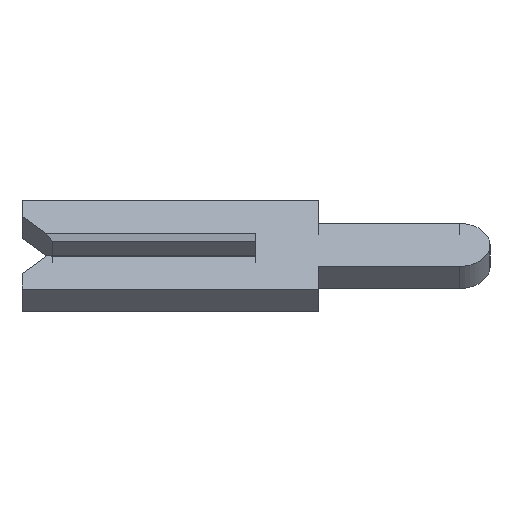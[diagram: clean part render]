
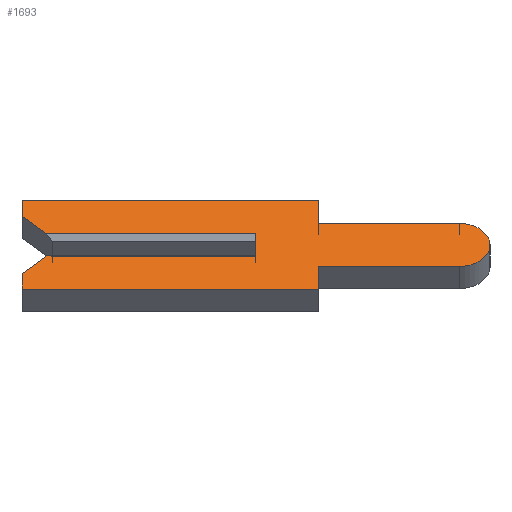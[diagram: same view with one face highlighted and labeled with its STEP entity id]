
A CAD part, left-side view. The second image highlights one B-rep face of the part: STEP entity #1693.
In plain terms, the highlighted face is planar.
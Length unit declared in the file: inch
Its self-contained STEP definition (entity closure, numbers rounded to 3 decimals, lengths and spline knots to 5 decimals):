
#19 = ORIENTED_EDGE ( 'NONE', *, *, #1580, .F. ) ;
#37 = LINE ( 'NONE', #1567, #1679 ) ;
#67 = ORIENTED_EDGE ( 'NONE', *, *, #1382, .F. ) ;
#69 = DIRECTION ( 'NONE',  ( 0., -1., 0. ) ) ;
#85 = VECTOR ( 'NONE', #317, 39.37008 ) ;
#98 = VERTEX_POINT ( 'NONE', #1309 ) ;
#99 = EDGE_CURVE ( 'NONE', #836, #1227, #289, .T. ) ;
#111 = VECTOR ( 'NONE', #650, 39.37008 ) ;
#124 = AXIS2_PLACEMENT_3D ( 'NONE', #1443, #1590, #241 ) ;
#133 = LINE ( 'NONE', #890, #406 ) ;
#152 = VECTOR ( 'NONE', #379, 39.37008 ) ;
#157 = CARTESIAN_POINT ( 'NONE',  ( -0.01, 0.15, -0.04 ) ) ;
#184 = LINE ( 'NONE', #938, #1361 ) ;
#218 = CARTESIAN_POINT ( 'NONE',  ( -0.01, 0.15, 0.04 ) ) ;
#241 = DIRECTION ( 'NONE',  ( 0., 0., -1. ) ) ;
#289 = LINE ( 'NONE', #1005, #1792 ) ;
#302 = VERTEX_POINT ( 'NONE', #1353 ) ;
#317 = DIRECTION ( 'NONE',  ( 0., 1., 0. ) ) ;
#320 = LINE ( 'NONE', #501, #973 ) ;
#353 = VERTEX_POINT ( 'NONE', #1051 ) ;
#359 = AXIS2_PLACEMENT_3D ( 'NONE', #1277, #968, #1577 ) ;
#379 = DIRECTION ( 'NONE',  ( 0., 0., 1. ) ) ;
#406 = VECTOR ( 'NONE', #440, 39.37008 ) ;
#440 = DIRECTION ( 'NONE',  ( 0., 1., 0. ) ) ;
#443 = CARTESIAN_POINT ( 'NONE',  ( -0.01, 0., -0.01 ) ) ;
#451 = LINE ( 'NONE', #1398, #1616 ) ;
#463 = EDGE_CURVE ( 'NONE', #1611, #98, #719, .T. ) ;
#493 = CARTESIAN_POINT ( 'NONE',  ( -0.01, -0.04, 0.0195 ) ) ;
#495 = LINE ( 'NONE', #986, #1040 ) ;
#501 = CARTESIAN_POINT ( 'NONE',  ( -0.01, 0.1305, 0.0065 ) ) ;
#518 = DIRECTION ( 'NONE',  ( 0., 0., 1. ) ) ;
#536 = DIRECTION ( 'NONE',  ( 0., -0.707, 0.707 ) ) ;
#548 = ORIENTED_EDGE ( 'NONE', *, *, #99, .F. ) ;
#575 = LINE ( 'NONE', #1581, #152 ) ;
#592 = VERTEX_POINT ( 'NONE', #443 ) ;
#613 = VERTEX_POINT ( 'NONE', #1502 ) ;
#614 = EDGE_CURVE ( 'NONE', #613, #836, #133, .T. ) ;
#625 = ORIENTED_EDGE ( 'NONE', *, *, #871, .F. ) ;
#633 = EDGE_CURVE ( 'NONE', #302, #1157, #184, .T. ) ;
#650 = DIRECTION ( 'NONE',  ( 0., -1., 0. ) ) ;
#671 = CARTESIAN_POINT ( 'NONE',  ( -0.01, 0., 0.01 ) ) ;
#712 = ORIENTED_EDGE ( 'NONE', *, *, #1259, .F. ) ;
#719 = LINE ( 'NONE', #1821, #1882 ) ;
#767 = CARTESIAN_POINT ( 'NONE',  ( -0.01, -0.04, 0.0195 ) ) ;
#768 = EDGE_CURVE ( 'NONE', #1324, #1337, #451, .T. ) ;
#801 = VECTOR ( 'NONE', #536, 39.37008 ) ;
#802 = VERTEX_POINT ( 'NONE', #1521 ) ;
#816 = CARTESIAN_POINT ( 'NONE',  ( -0.01, -0.04, 0.04 ) ) ;
#834 = CARTESIAN_POINT ( 'NONE',  ( -0.01, 0.1305, -0.0065 ) ) ;
#836 = VERTEX_POINT ( 'NONE', #1085 ) ;
#837 = ORIENTED_EDGE ( 'NONE', *, *, #633, .T. ) ;
#856 = CARTESIAN_POINT ( 'NONE',  ( -0.01, 0.134, -0.01 ) ) ;
#871 = EDGE_CURVE ( 'NONE', #1227, #1611, #1757, .T. ) ;
#890 = CARTESIAN_POINT ( 'NONE',  ( -0.01, -0.04, -0.0195 ) ) ;
#915 = DIRECTION ( 'NONE',  ( 0., 0., -1. ) ) ;
#919 = FACE_OUTER_BOUND ( 'NONE', #1469, .T. ) ;
#938 = CARTESIAN_POINT ( 'NONE',  ( -0.01, 0.15, 0.01 ) ) ;
#968 = DIRECTION ( 'NONE',  ( 1., 0., 0. ) ) ;
#973 = VECTOR ( 'NONE', #1549, 39.37008 ) ;
#986 = CARTESIAN_POINT ( 'NONE',  ( -0.01, -0.1305, -0.01 ) ) ;
#1005 = CARTESIAN_POINT ( 'NONE',  ( -0.01, -0.04, -0.04 ) ) ;
#1016 = ORIENTED_EDGE ( 'NONE', *, *, #1139, .F. ) ;
#1040 = VECTOR ( 'NONE', #69, 39.37008 ) ;
#1043 = ORIENTED_EDGE ( 'NONE', *, *, #1756, .F. ) ;
#1051 = CARTESIAN_POINT ( 'NONE',  ( -0.01, -0.1305, 0.0195 ) ) ;
#1070 = DIRECTION ( 'NONE',  ( 0., -1., 0. ) ) ;
#1073 = DIRECTION ( 'NONE',  ( 0., -1., 0. ) ) ;
#1074 = EDGE_CURVE ( 'NONE', #1337, #353, #1376, .T. ) ;
#1085 = CARTESIAN_POINT ( 'NONE',  ( -0.01, -0.04, -0.0195 ) ) ;
#1111 = ORIENTED_EDGE ( 'NONE', *, *, #1283, .F. ) ;
#1139 = EDGE_CURVE ( 'NONE', #592, #1157, #37, .T. ) ;
#1146 = PLANE ( 'NONE',  #124 ) ;
#1157 = VERTEX_POINT ( 'NONE', #671 ) ;
#1227 = VERTEX_POINT ( 'NONE', #1251 ) ;
#1236 = ORIENTED_EDGE ( 'NONE', *, *, #768, .F. ) ;
#1237 = ORIENTED_EDGE ( 'NONE', *, *, #614, .F. ) ;
#1251 = CARTESIAN_POINT ( 'NONE',  ( -0.01, -0.04, -0.04 ) ) ;
#1259 = EDGE_CURVE ( 'NONE', #353, #613, #1525, .T. ) ;
#1277 = CARTESIAN_POINT ( 'NONE',  ( -0.01, -0.1305, 0. ) ) ;
#1283 = EDGE_CURVE ( 'NONE', #1465, #1324, #1485, .T. ) ;
#1303 = ORIENTED_EDGE ( 'NONE', *, *, #1538, .F. ) ;
#1309 = CARTESIAN_POINT ( 'NONE',  ( -0.01, 0.15, -0.026 ) ) ;
#1317 = DIRECTION ( 'NONE',  ( 0., 0., -1. ) ) ;
#1324 = VERTEX_POINT ( 'NONE', #816 ) ;
#1337 = VERTEX_POINT ( 'NONE', #493 ) ;
#1353 = CARTESIAN_POINT ( 'NONE',  ( -0.01, 0.134, 0.01 ) ) ;
#1361 = VECTOR ( 'NONE', #1070, 39.37008 ) ;
#1376 = LINE ( 'NONE', #767, #1785 ) ;
#1382 = EDGE_CURVE ( 'NONE', #302, #802, #320, .T. ) ;
#1398 = CARTESIAN_POINT ( 'NONE',  ( -0.01, -0.04, 0.04 ) ) ;
#1443 = CARTESIAN_POINT ( 'NONE',  ( -0.01, -0.1305, 0. ) ) ;
#1465 = VERTEX_POINT ( 'NONE', #1871 ) ;
#1469 = EDGE_LOOP ( 'NONE', ( #837, #1016, #19, #1043, #1717, #625, #548, #1237, #712, #1598, #1236, #1111, #1303, #67 ) ) ;
#1485 = LINE ( 'NONE', #218, #111 ) ;
#1502 = CARTESIAN_POINT ( 'NONE',  ( -0.01, -0.1305, -0.0195 ) ) ;
#1521 = CARTESIAN_POINT ( 'NONE',  ( -0.01, 0.15, 0.026 ) ) ;
#1525 = CIRCLE ( 'NONE', #359, 0.0195 ) ;
#1538 = EDGE_CURVE ( 'NONE', #802, #1465, #575, .T. ) ;
#1549 = DIRECTION ( 'NONE',  ( 0., 0.707, 0.707 ) ) ;
#1553 = LINE ( 'NONE', #834, #801 ) ;
#1567 = CARTESIAN_POINT ( 'NONE',  ( -0.01, 0., 0.0065 ) ) ;
#1569 = VERTEX_POINT ( 'NONE', #856 ) ;
#1577 = DIRECTION ( 'NONE',  ( 0., 0., -1. ) ) ;
#1580 = EDGE_CURVE ( 'NONE', #1569, #592, #495, .T. ) ;
#1581 = CARTESIAN_POINT ( 'NONE',  ( -0.01, 0.15, 0.026 ) ) ;
#1590 = DIRECTION ( 'NONE',  ( 1., 0., 0. ) ) ;
#1598 = ORIENTED_EDGE ( 'NONE', *, *, #1074, .F. ) ;
#1611 = VERTEX_POINT ( 'NONE', #1895 ) ;
#1616 = VECTOR ( 'NONE', #915, 39.37008 ) ;
#1679 = VECTOR ( 'NONE', #518, 39.37008 ) ;
#1693 = ADVANCED_FACE ( 'NONE', ( #919 ), #1146, .F. ) ;
#1717 = ORIENTED_EDGE ( 'NONE', *, *, #463, .F. ) ;
#1756 = EDGE_CURVE ( 'NONE', #98, #1569, #1553, .T. ) ;
#1757 = LINE ( 'NONE', #157, #85 ) ;
#1785 = VECTOR ( 'NONE', #1073, 39.37008 ) ;
#1792 = VECTOR ( 'NONE', #1317, 39.37008 ) ;
#1812 = DIRECTION ( 'NONE',  ( 0., 0., 1. ) ) ;
#1821 = CARTESIAN_POINT ( 'NONE',  ( -0.01, 0.15, -0.026 ) ) ;
#1871 = CARTESIAN_POINT ( 'NONE',  ( -0.01, 0.15, 0.04 ) ) ;
#1882 = VECTOR ( 'NONE', #1812, 39.37008 ) ;
#1895 = CARTESIAN_POINT ( 'NONE',  ( -0.01, 0.15, -0.04 ) ) ;
